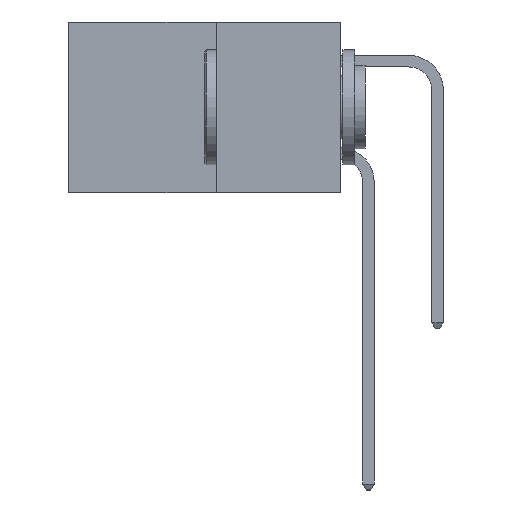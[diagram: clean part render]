
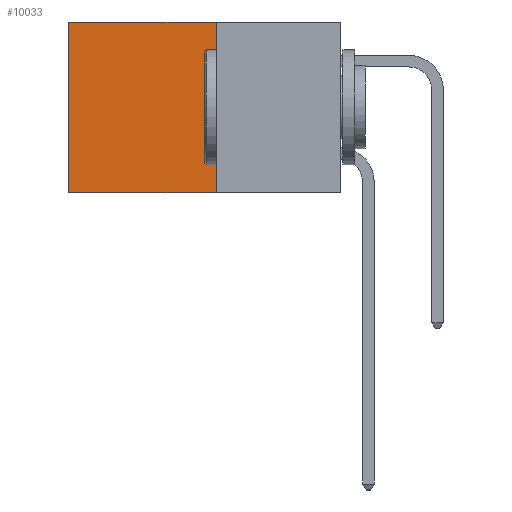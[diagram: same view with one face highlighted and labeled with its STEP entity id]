
A CAD part, left-side view. The second image highlights one B-rep face of the part: STEP entity #10033.
In plain terms, the highlighted planar face has unit normal (-1, 0, 0).
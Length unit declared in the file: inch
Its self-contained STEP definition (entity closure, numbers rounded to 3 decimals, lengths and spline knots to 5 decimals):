
#159 = EDGE_CURVE ( 'NONE', #6962, #3885, #11533, .T. ) ;
#241 = VECTOR ( 'NONE', #5191, 39.37008 ) ;
#549 = DIRECTION ( 'NONE',  ( 0., 0., -1. ) ) ;
#820 = EDGE_CURVE ( 'NONE', #11522, #6962, #5981, .T. ) ;
#928 = CARTESIAN_POINT ( 'NONE',  ( 0.277, 0.27, -0.37 ) ) ;
#982 = DIRECTION ( 'NONE',  ( 1., 0., 0. ) ) ;
#1014 = CARTESIAN_POINT ( 'NONE',  ( 0.277, 0.27, 0. ) ) ;
#1016 = CARTESIAN_POINT ( 'NONE',  ( 0.277, 0.59, -0.37 ) ) ;
#1238 = DIRECTION ( 'NONE',  ( 0., 0., -1. ) ) ;
#2124 = CARTESIAN_POINT ( 'NONE',  ( 0.277, 0.59, 0. ) ) ;
#2312 = CARTESIAN_POINT ( 'NONE',  ( 0.277, 0.27, -0.37 ) ) ;
#2903 = EDGE_CURVE ( 'NONE', #11522, #4128, #10974, .T. ) ;
#3885 = VERTEX_POINT ( 'NONE', #4704 ) ;
#4128 = VERTEX_POINT ( 'NONE', #2124 ) ;
#4208 = EDGE_CURVE ( 'NONE', #4128, #3885, #6535, .T. ) ;
#4704 = CARTESIAN_POINT ( 'NONE',  ( 0.277, 0.59, -0.37 ) ) ;
#5191 = DIRECTION ( 'NONE',  ( 0., 1., 0. ) ) ;
#5981 = LINE ( 'NONE', #11571, #12609 ) ;
#6535 = LINE ( 'NONE', #1016, #11454 ) ;
#6817 = ORIENTED_EDGE ( 'NONE', *, *, #820, .F. ) ;
#6962 = VERTEX_POINT ( 'NONE', #2312 ) ;
#7188 = FACE_OUTER_BOUND ( 'NONE', #11762, .T. ) ;
#7231 = CARTESIAN_POINT ( 'NONE',  ( 0.277, 0.27, 0. ) ) ;
#8495 = DIRECTION ( 'NONE',  ( 0., 0., -1. ) ) ;
#9111 = ORIENTED_EDGE ( 'NONE', *, *, #4208, .T. ) ;
#9228 = VECTOR ( 'NONE', #12906, 39.37008 ) ;
#9397 = ORIENTED_EDGE ( 'NONE', *, *, #2903, .T. ) ;
#10033 = ADVANCED_FACE ( 'NONE', ( #7188 ), #11954, .F. ) ;
#10974 = LINE ( 'NONE', #7231, #241 ) ;
#11434 = ORIENTED_EDGE ( 'NONE', *, *, #159, .F. ) ;
#11454 = VECTOR ( 'NONE', #1238, 39.37008 ) ;
#11522 = VERTEX_POINT ( 'NONE', #1014 ) ;
#11533 = LINE ( 'NONE', #11667, #9228 ) ;
#11571 = CARTESIAN_POINT ( 'NONE',  ( 0.277, 0.27, -0.37 ) ) ;
#11667 = CARTESIAN_POINT ( 'NONE',  ( 0.277, 0.27, -0.37 ) ) ;
#11762 = EDGE_LOOP ( 'NONE', ( #9111, #11434, #6817, #9397 ) ) ;
#11794 = AXIS2_PLACEMENT_3D ( 'NONE', #928, #982, #8495 ) ;
#11954 = PLANE ( 'NONE',  #11794 ) ;
#12609 = VECTOR ( 'NONE', #549, 39.37008 ) ;
#12906 = DIRECTION ( 'NONE',  ( 0., 1., 0. ) ) ;
